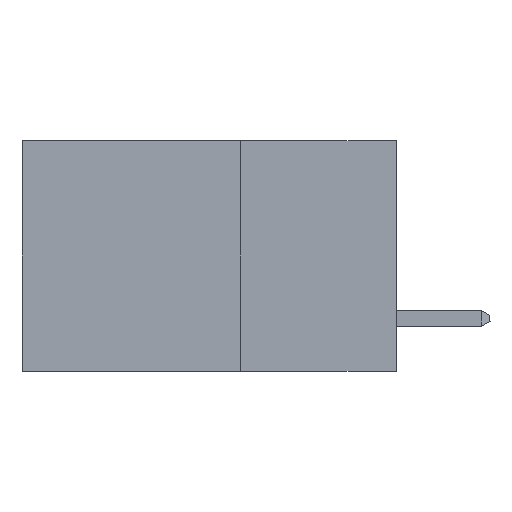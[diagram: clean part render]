
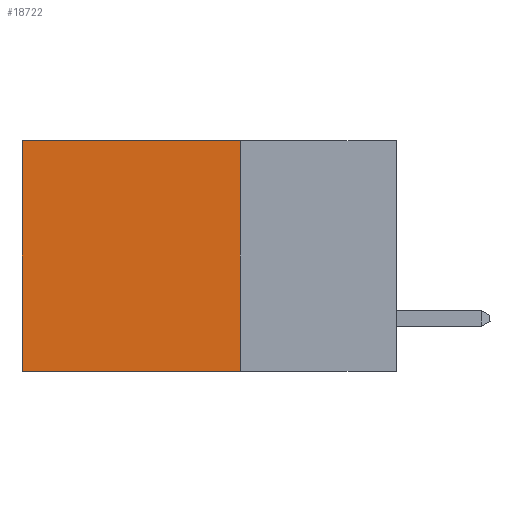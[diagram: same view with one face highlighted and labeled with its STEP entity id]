
A CAD part, left-side view. The second image highlights one B-rep face of the part: STEP entity #18722.
In plain terms, the highlighted planar face has unit normal (-1, 0, 0).
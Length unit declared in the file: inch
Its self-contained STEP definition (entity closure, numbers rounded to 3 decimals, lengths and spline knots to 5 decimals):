
#955 = ORIENTED_EDGE ( 'NONE', *, *, #24986, .F. ) ;
#1117 = CARTESIAN_POINT ( 'NONE',  ( 0.298, 0.6, 0. ) ) ;
#1516 = DIRECTION ( 'NONE',  ( 0., 1., 0. ) ) ;
#1861 = PLANE ( 'NONE',  #18672 ) ;
#2592 = DIRECTION ( 'NONE',  ( 0., 1., 0. ) ) ;
#4810 = CARTESIAN_POINT ( 'NONE',  ( 0.298, 0.25, 0. ) ) ;
#4862 = VERTEX_POINT ( 'NONE', #22741 ) ;
#4973 = VECTOR ( 'NONE', #1516, 39.37008 ) ;
#5905 = DIRECTION ( 'NONE',  ( 0., 0., -1. ) ) ;
#6161 = ORIENTED_EDGE ( 'NONE', *, *, #20008, .T. ) ;
#6204 = CARTESIAN_POINT ( 'NONE',  ( 0.298, 0.6, 0. ) ) ;
#6279 = EDGE_LOOP ( 'NONE', ( #8111, #10546, #955, #6161 ) ) ;
#7978 = LINE ( 'NONE', #1117, #12599 ) ;
#8082 = VERTEX_POINT ( 'NONE', #21739 ) ;
#8111 = ORIENTED_EDGE ( 'NONE', *, *, #25100, .T. ) ;
#8892 = LINE ( 'NONE', #10450, #18828 ) ;
#10450 = CARTESIAN_POINT ( 'NONE',  ( 0.298, 0.25, 0. ) ) ;
#10546 = ORIENTED_EDGE ( 'NONE', *, *, #24016, .F. ) ;
#11060 = VECTOR ( 'NONE', #22632, 39.37008 ) ;
#11412 = CARTESIAN_POINT ( 'NONE',  ( 0.298, 0.25, -0.37 ) ) ;
#12599 = VECTOR ( 'NONE', #19054, 39.37008 ) ;
#15701 = CARTESIAN_POINT ( 'NONE',  ( 0.298, 0.25, 0. ) ) ;
#16832 = VERTEX_POINT ( 'NONE', #6204 ) ;
#17606 = CARTESIAN_POINT ( 'NONE',  ( 0.298, 0.25, 0. ) ) ;
#17706 = DIRECTION ( 'NONE',  ( 1., 0., 0. ) ) ;
#18672 = AXIS2_PLACEMENT_3D ( 'NONE', #15701, #17706, #5905 ) ;
#18722 = ADVANCED_FACE ( 'NONE', ( #24609 ), #1861, .F. ) ;
#18828 = VECTOR ( 'NONE', #2592, 39.37008 ) ;
#19054 = DIRECTION ( 'NONE',  ( 0., 0., -1. ) ) ;
#20008 = EDGE_CURVE ( 'NONE', #22561, #16832, #8892, .T. ) ;
#21584 = LINE ( 'NONE', #4810, #11060 ) ;
#21739 = CARTESIAN_POINT ( 'NONE',  ( 0.298, 0.25, -0.37 ) ) ;
#22561 = VERTEX_POINT ( 'NONE', #17606 ) ;
#22632 = DIRECTION ( 'NONE',  ( 0., 0., -1. ) ) ;
#22741 = CARTESIAN_POINT ( 'NONE',  ( 0.298, 0.6, -0.37 ) ) ;
#24016 = EDGE_CURVE ( 'NONE', #8082, #4862, #25378, .T. ) ;
#24609 = FACE_OUTER_BOUND ( 'NONE', #6279, .T. ) ;
#24986 = EDGE_CURVE ( 'NONE', #22561, #8082, #21584, .T. ) ;
#25100 = EDGE_CURVE ( 'NONE', #16832, #4862, #7978, .T. ) ;
#25378 = LINE ( 'NONE', #11412, #4973 ) ;
